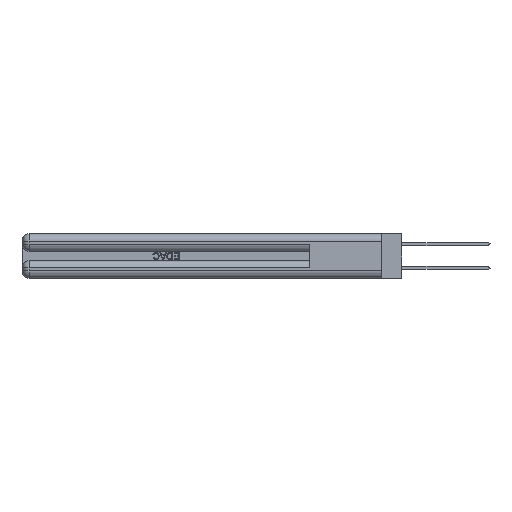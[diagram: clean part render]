
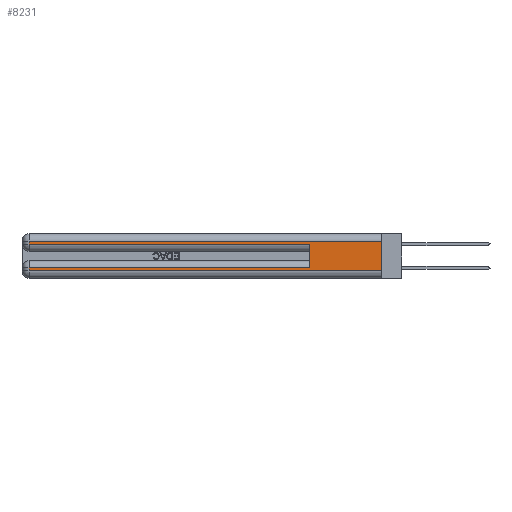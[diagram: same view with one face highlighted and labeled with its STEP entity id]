
A CAD part, left-side view. The second image highlights one B-rep face of the part: STEP entity #8231.
In plain terms, the highlighted planar face has unit normal (-1, 0, 0).
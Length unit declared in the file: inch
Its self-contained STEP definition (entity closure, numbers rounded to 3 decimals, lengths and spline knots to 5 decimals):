
#932 = DIRECTION ( 'NONE',  ( 1., 0., 0. ) ) ;
#1240 = CARTESIAN_POINT ( 'NONE',  ( 0., 0.6, 0.085 ) ) ;
#1442 = PLANE ( 'NONE',  #25854 ) ;
#1610 = CARTESIAN_POINT ( 'NONE',  ( 0., 0., 0.285 ) ) ;
#2937 = DIRECTION ( 'NONE',  ( 0., 0., -1. ) ) ;
#4328 = DIRECTION ( 'NONE',  ( 0., 0., 1. ) ) ;
#4523 = VECTOR ( 'NONE', #23426, 39.37008 ) ;
#5096 = DIRECTION ( 'NONE',  ( 0., -1., 0. ) ) ;
#5205 = EDGE_CURVE ( 'NONE', #19640, #10636, #29538, .T. ) ;
#5545 = ORIENTED_EDGE ( 'NONE', *, *, #25900, .T. ) ;
#7897 = VECTOR ( 'NONE', #4328, 39.37008 ) ;
#8174 = FACE_OUTER_BOUND ( 'NONE', #28470, .T. ) ;
#8231 = ADVANCED_FACE ( 'NONE', ( #8174 ), #1442, .F. ) ;
#8297 = VECTOR ( 'NONE', #2937, 39.37008 ) ;
#8591 = VERTEX_POINT ( 'NONE', #18401 ) ;
#9432 = ORIENTED_EDGE ( 'NONE', *, *, #23079, .T. ) ;
#10488 = VECTOR ( 'NONE', #26057, 39.37008 ) ;
#10636 = VERTEX_POINT ( 'NONE', #40277 ) ;
#11407 = CARTESIAN_POINT ( 'NONE',  ( 0., 2.94, 0.31 ) ) ;
#11753 = ORIENTED_EDGE ( 'NONE', *, *, #38066, .T. ) ;
#13850 = LINE ( 'NONE', #42675, #8297 ) ;
#16600 = CARTESIAN_POINT ( 'NONE',  ( 0., 0., 0.06 ) ) ;
#17684 = VECTOR ( 'NONE', #48767, 39.37008 ) ;
#17882 = EDGE_CURVE ( 'NONE', #26711, #26315, #31824, .T. ) ;
#18118 = EDGE_CURVE ( 'NONE', #26984, #8591, #13850, .T. ) ;
#18401 = CARTESIAN_POINT ( 'NONE',  ( 0., 2.94, 0.285 ) ) ;
#19640 = VERTEX_POINT ( 'NONE', #1240 ) ;
#20300 = EDGE_CURVE ( 'NONE', #34331, #26315, #29138, .T. ) ;
#20775 = CARTESIAN_POINT ( 'NONE',  ( 0., 0., 0.31 ) ) ;
#22186 = DIRECTION ( 'NONE',  ( 0., 0., -1. ) ) ;
#23079 = EDGE_CURVE ( 'NONE', #26711, #26984, #39939, .T. ) ;
#23426 = DIRECTION ( 'NONE',  ( 0., 0., -1. ) ) ;
#24993 = DIRECTION ( 'NONE',  ( 0., 0., -1. ) ) ;
#25393 = ORIENTED_EDGE ( 'NONE', *, *, #20300, .T. ) ;
#25644 = CARTESIAN_POINT ( 'NONE',  ( 0., 2.94, 0.37 ) ) ;
#25753 = LINE ( 'NONE', #25644, #30071 ) ;
#25854 = AXIS2_PLACEMENT_3D ( 'NONE', #32624, #932, #24993 ) ;
#25900 = EDGE_CURVE ( 'NONE', #8591, #10636, #37740, .T. ) ;
#26057 = DIRECTION ( 'NONE',  ( 0., 1., 0. ) ) ;
#26315 = VERTEX_POINT ( 'NONE', #39453 ) ;
#26711 = VERTEX_POINT ( 'NONE', #45143 ) ;
#26984 = VERTEX_POINT ( 'NONE', #11407 ) ;
#27216 = VECTOR ( 'NONE', #5096, 39.37008 ) ;
#27529 = CARTESIAN_POINT ( 'NONE',  ( 0., 0.6, 0.145 ) ) ;
#28470 = EDGE_LOOP ( 'NONE', ( #34218, #9432, #31490, #5545, #29361, #11753, #51036, #25393 ) ) ;
#28843 = EDGE_CURVE ( 'NONE', #44128, #34331, #25753, .T. ) ;
#29138 = LINE ( 'NONE', #16600, #45834 ) ;
#29361 = ORIENTED_EDGE ( 'NONE', *, *, #5205, .F. ) ;
#29538 = LINE ( 'NONE', #27529, #7897 ) ;
#30071 = VECTOR ( 'NONE', #22186, 39.37008 ) ;
#30379 = CARTESIAN_POINT ( 'NONE',  ( 0., 0., 0.37 ) ) ;
#31490 = ORIENTED_EDGE ( 'NONE', *, *, #18118, .T. ) ;
#31824 = LINE ( 'NONE', #30379, #4523 ) ;
#32624 = CARTESIAN_POINT ( 'NONE',  ( 0., 0., 0.37 ) ) ;
#34218 = ORIENTED_EDGE ( 'NONE', *, *, #17882, .F. ) ;
#34331 = VERTEX_POINT ( 'NONE', #43843 ) ;
#34958 = CARTESIAN_POINT ( 'NONE',  ( 0., 2.94, 0.085 ) ) ;
#37740 = LINE ( 'NONE', #1610, #27216 ) ;
#38066 = EDGE_CURVE ( 'NONE', #19640, #44128, #42622, .T. ) ;
#39453 = CARTESIAN_POINT ( 'NONE',  ( 0., 0., 0.06 ) ) ;
#39939 = LINE ( 'NONE', #20775, #17684 ) ;
#40107 = DIRECTION ( 'NONE',  ( 0., -1., 0. ) ) ;
#40277 = CARTESIAN_POINT ( 'NONE',  ( 0., 0.6, 0.285 ) ) ;
#42622 = LINE ( 'NONE', #45731, #10488 ) ;
#42675 = CARTESIAN_POINT ( 'NONE',  ( 0., 2.94, 0.37 ) ) ;
#43843 = CARTESIAN_POINT ( 'NONE',  ( 0., 2.94, 0.06 ) ) ;
#44128 = VERTEX_POINT ( 'NONE', #34958 ) ;
#45143 = CARTESIAN_POINT ( 'NONE',  ( 0., 0., 0.31 ) ) ;
#45731 = CARTESIAN_POINT ( 'NONE',  ( 0., 0., 0.085 ) ) ;
#45834 = VECTOR ( 'NONE', #40107, 39.37008 ) ;
#48767 = DIRECTION ( 'NONE',  ( 0., 1., 0. ) ) ;
#51036 = ORIENTED_EDGE ( 'NONE', *, *, #28843, .T. ) ;
